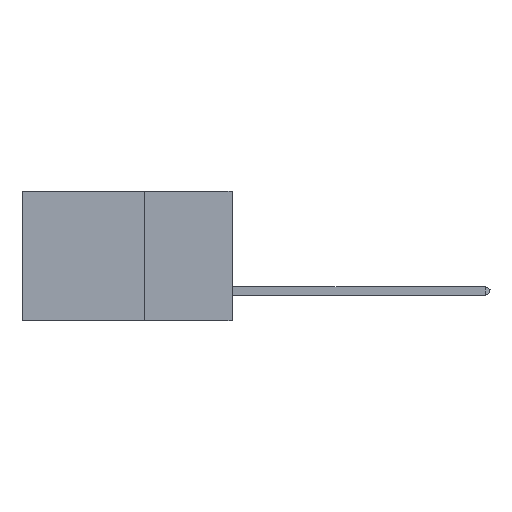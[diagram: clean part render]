
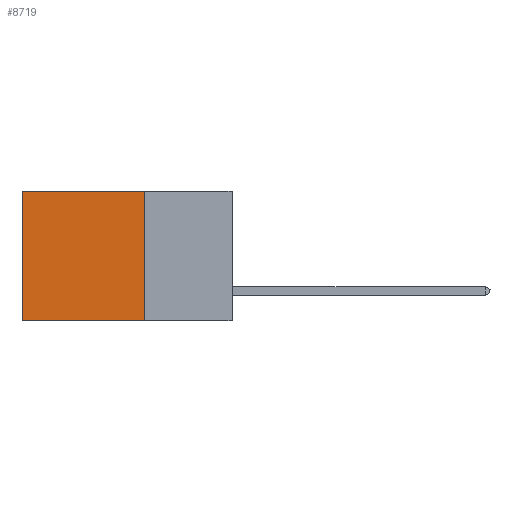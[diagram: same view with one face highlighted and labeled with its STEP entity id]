
A CAD part, left-side view. The second image highlights one B-rep face of the part: STEP entity #8719.
In plain terms, the highlighted planar face has unit normal (-1, 0, 0).
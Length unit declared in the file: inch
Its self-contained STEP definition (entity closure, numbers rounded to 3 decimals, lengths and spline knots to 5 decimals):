
#1821 = DIRECTION ( 'NONE',  ( 0., 1., 0. ) ) ;
#4217 = EDGE_CURVE ( 'NONE', #25723, #30453, #4485, .T. ) ;
#4485 = LINE ( 'NONE', #20508, #24918 ) ;
#4976 = CARTESIAN_POINT ( 'NONE',  ( 0.2875, 0.25, -0.37 ) ) ;
#6544 = CARTESIAN_POINT ( 'NONE',  ( 0.2875, 0.6, 0. ) ) ;
#7086 = ORIENTED_EDGE ( 'NONE', *, *, #30147, .T. ) ;
#8544 = PLANE ( 'NONE',  #19544 ) ;
#8719 = ADVANCED_FACE ( 'NONE', ( #14433 ), #8544, .F. ) ;
#11264 = VERTEX_POINT ( 'NONE', #17162 ) ;
#14433 = FACE_OUTER_BOUND ( 'NONE', #33785, .T. ) ;
#14807 = DIRECTION ( 'NONE',  ( 0., 0., -1. ) ) ;
#15955 = VECTOR ( 'NONE', #14807, 39.37008 ) ;
#17162 = CARTESIAN_POINT ( 'NONE',  ( 0.2875, 0.6, -0.37 ) ) ;
#17284 = CARTESIAN_POINT ( 'NONE',  ( 0.2875, 0.25, 0. ) ) ;
#19099 = CARTESIAN_POINT ( 'NONE',  ( 0.2875, 0.25, 0. ) ) ;
#19544 = AXIS2_PLACEMENT_3D ( 'NONE', #17284, #35066, #20325 ) ;
#20053 = LINE ( 'NONE', #6544, #15955 ) ;
#20325 = DIRECTION ( 'NONE',  ( 0., 0., -1. ) ) ;
#20416 = EDGE_CURVE ( 'NONE', #30453, #11264, #36687, .T. ) ;
#20508 = CARTESIAN_POINT ( 'NONE',  ( 0.2875, 0.25, 0. ) ) ;
#21212 = VECTOR ( 'NONE', #24134, 39.37008 ) ;
#22170 = LINE ( 'NONE', #19099, #24450 ) ;
#24134 = DIRECTION ( 'NONE',  ( 0., 1., 0. ) ) ;
#24450 = VECTOR ( 'NONE', #1821, 39.37008 ) ;
#24817 = CARTESIAN_POINT ( 'NONE',  ( 0.2875, 0.6, 0. ) ) ;
#24918 = VECTOR ( 'NONE', #29367, 39.37008 ) ;
#25723 = VERTEX_POINT ( 'NONE', #34106 ) ;
#26918 = CARTESIAN_POINT ( 'NONE',  ( 0.2875, 0.25, -0.37 ) ) ;
#29367 = DIRECTION ( 'NONE',  ( 0., 0., -1. ) ) ;
#30147 = EDGE_CURVE ( 'NONE', #35150, #11264, #20053, .T. ) ;
#30453 = VERTEX_POINT ( 'NONE', #4976 ) ;
#30680 = ORIENTED_EDGE ( 'NONE', *, *, #32331, .T. ) ;
#32331 = EDGE_CURVE ( 'NONE', #25723, #35150, #22170, .T. ) ;
#33785 = EDGE_LOOP ( 'NONE', ( #7086, #35793, #34893, #30680 ) ) ;
#34106 = CARTESIAN_POINT ( 'NONE',  ( 0.2875, 0.25, 0. ) ) ;
#34893 = ORIENTED_EDGE ( 'NONE', *, *, #4217, .F. ) ;
#35066 = DIRECTION ( 'NONE',  ( 1., 0., 0. ) ) ;
#35150 = VERTEX_POINT ( 'NONE', #24817 ) ;
#35793 = ORIENTED_EDGE ( 'NONE', *, *, #20416, .F. ) ;
#36687 = LINE ( 'NONE', #26918, #21212 ) ;
